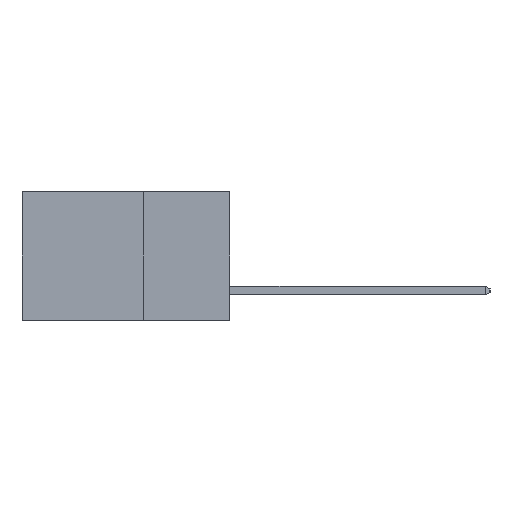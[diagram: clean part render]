
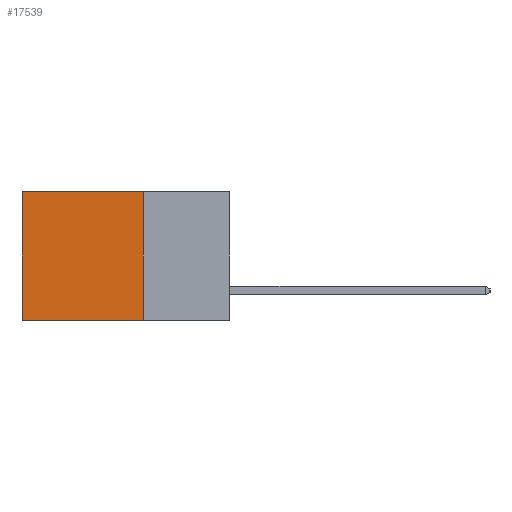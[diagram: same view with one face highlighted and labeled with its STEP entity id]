
A CAD part, left-side view. The second image highlights one B-rep face of the part: STEP entity #17539.
In plain terms, the highlighted planar face has unit normal (-1, 0, 0).
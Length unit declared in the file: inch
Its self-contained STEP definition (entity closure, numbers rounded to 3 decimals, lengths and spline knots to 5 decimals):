
#245 = AXIS2_PLACEMENT_3D ( 'NONE', #14872, #4761, #16549 ) ;
#889 = EDGE_CURVE ( 'NONE', #9889, #20504, #2996, .T. ) ;
#1028 = FACE_OUTER_BOUND ( 'NONE', #13012, .T. ) ;
#1323 = PLANE ( 'NONE',  #245 ) ;
#1415 = ORIENTED_EDGE ( 'NONE', *, *, #11765, .T. ) ;
#1674 = LINE ( 'NONE', #8458, #15704 ) ;
#2298 = CARTESIAN_POINT ( 'NONE',  ( 0.298, 0.25, 0. ) ) ;
#2996 = LINE ( 'NONE', #5862, #15945 ) ;
#4003 = DIRECTION ( 'NONE',  ( 0., 1., 0. ) ) ;
#4669 = DIRECTION ( 'NONE',  ( 0., 0., -1. ) ) ;
#4761 = DIRECTION ( 'NONE',  ( 1., 0., 0. ) ) ;
#5862 = CARTESIAN_POINT ( 'NONE',  ( 0.298, 0.25, 0. ) ) ;
#6166 = CARTESIAN_POINT ( 'NONE',  ( 0.298, 0.25, 0. ) ) ;
#7668 = DIRECTION ( 'NONE',  ( 0., 0., -1. ) ) ;
#8458 = CARTESIAN_POINT ( 'NONE',  ( 0.298, 0.25, -0.37 ) ) ;
#8512 = VECTOR ( 'NONE', #7668, 39.37008 ) ;
#9083 = ORIENTED_EDGE ( 'NONE', *, *, #11027, .T. ) ;
#9889 = VERTEX_POINT ( 'NONE', #6166 ) ;
#9927 = CARTESIAN_POINT ( 'NONE',  ( 0.298, 0.6, 0. ) ) ;
#10140 = LINE ( 'NONE', #2298, #14622 ) ;
#11027 = EDGE_CURVE ( 'NONE', #9889, #18272, #10140, .T. ) ;
#11687 = ORIENTED_EDGE ( 'NONE', *, *, #889, .F. ) ;
#11765 = EDGE_CURVE ( 'NONE', #18272, #17516, #18487, .T. ) ;
#13012 = EDGE_LOOP ( 'NONE', ( #1415, #15569, #11687, #9083 ) ) ;
#14622 = VECTOR ( 'NONE', #4003, 39.37008 ) ;
#14872 = CARTESIAN_POINT ( 'NONE',  ( 0.298, 0.25, 0. ) ) ;
#15569 = ORIENTED_EDGE ( 'NONE', *, *, #15885, .F. ) ;
#15704 = VECTOR ( 'NONE', #20157, 39.37008 ) ;
#15885 = EDGE_CURVE ( 'NONE', #20504, #17516, #1674, .T. ) ;
#15945 = VECTOR ( 'NONE', #4669, 39.37008 ) ;
#16483 = CARTESIAN_POINT ( 'NONE',  ( 0.298, 0.6, -0.37 ) ) ;
#16549 = DIRECTION ( 'NONE',  ( 0., 0., -1. ) ) ;
#17516 = VERTEX_POINT ( 'NONE', #16483 ) ;
#17539 = ADVANCED_FACE ( 'NONE', ( #1028 ), #1323, .F. ) ;
#18272 = VERTEX_POINT ( 'NONE', #9927 ) ;
#18487 = LINE ( 'NONE', #19367, #8512 ) ;
#19367 = CARTESIAN_POINT ( 'NONE',  ( 0.298, 0.6, 0. ) ) ;
#20157 = DIRECTION ( 'NONE',  ( 0., 1., 0. ) ) ;
#20258 = CARTESIAN_POINT ( 'NONE',  ( 0.298, 0.25, -0.37 ) ) ;
#20504 = VERTEX_POINT ( 'NONE', #20258 ) ;
